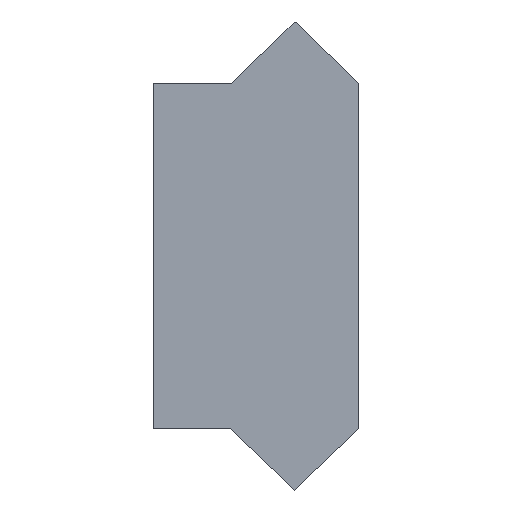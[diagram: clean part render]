
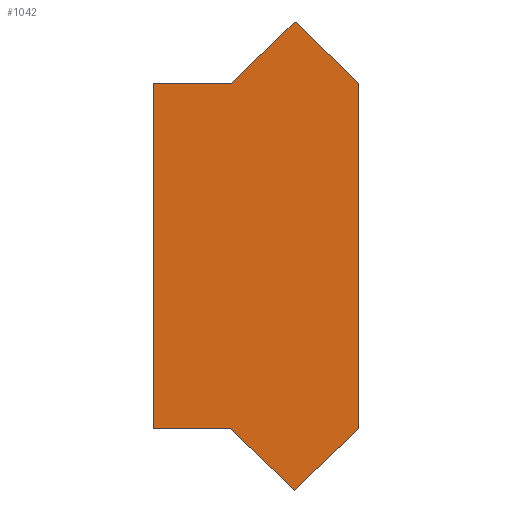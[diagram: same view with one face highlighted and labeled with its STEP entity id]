
A CAD part, front view. The second image highlights one B-rep face of the part: STEP entity #1042.
In plain terms, the highlighted planar face has unit normal (0, -1, 0).
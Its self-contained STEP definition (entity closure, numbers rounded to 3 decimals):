
#72=PLANE('',#1111);
#126=FACE_OUTER_BOUND('',#184,.T.);
#184=EDGE_LOOP('',(#977,#978,#979,#980,#981,#982,#983,#984));
#216=LINE('',#1477,#348);
#219=LINE('',#1482,#351);
#249=LINE('',#1544,#381);
#265=LINE('',#1577,#397);
#282=LINE('',#1607,#414);
#312=LINE('',#1666,#444);
#314=LINE('',#1670,#446);
#316=LINE('',#1673,#448);
#348=VECTOR('',#1196,10.);
#351=VECTOR('',#1201,10.);
#381=VECTOR('',#1243,10.);
#397=VECTOR('',#1269,10.);
#414=VECTOR('',#1300,10.);
#444=VECTOR('',#1370,10.);
#446=VECTOR('',#1374,10.);
#448=VECTOR('',#1378,10.);
#496=VERTEX_POINT('',#1475);
#497=VERTEX_POINT('',#1476);
#498=VERTEX_POINT('',#1481);
#523=VERTEX_POINT('',#1542);
#524=VERTEX_POINT('',#1543);
#536=VERTEX_POINT('',#1576);
#551=VERTEX_POINT('',#1665);
#552=VERTEX_POINT('',#1669);
#596=EDGE_CURVE('',#496,#497,#216,.T.);
#599=EDGE_CURVE('',#497,#498,#219,.T.);
#629=EDGE_CURVE('',#523,#524,#249,.T.);
#645=EDGE_CURVE('',#524,#536,#265,.T.);
#662=EDGE_CURVE('',#536,#498,#282,.T.);
#692=EDGE_CURVE('',#523,#551,#312,.T.);
#694=EDGE_CURVE('',#551,#552,#314,.T.);
#696=EDGE_CURVE('',#552,#496,#316,.T.);
#977=ORIENTED_EDGE('',*,*,#692,.T.);
#978=ORIENTED_EDGE('',*,*,#694,.T.);
#979=ORIENTED_EDGE('',*,*,#696,.T.);
#980=ORIENTED_EDGE('',*,*,#596,.T.);
#981=ORIENTED_EDGE('',*,*,#599,.T.);
#982=ORIENTED_EDGE('',*,*,#662,.F.);
#983=ORIENTED_EDGE('',*,*,#645,.F.);
#984=ORIENTED_EDGE('',*,*,#629,.F.);
#1042=ADVANCED_FACE('',(#126),#72,.T.);
#1111=AXIS2_PLACEMENT_3D('',#1674,#1379,#1380);
#1196=DIRECTION('',(1.,0.,0.));
#1201=DIRECTION('',(0.725,0.,-0.689));
#1243=DIRECTION('',(0.722,0.,-0.692));
#1269=DIRECTION('',(0.,0.,-1.));
#1300=DIRECTION('',(-0.726,0.,-0.688));
#1370=DIRECTION('',(-0.723,0.,-0.691));
#1374=DIRECTION('',(-1.,0.,0.));
#1378=DIRECTION('',(0.,0.,-1.));
#1379=DIRECTION('center_axis',(0.,-1.,0.));
#1380=DIRECTION('ref_axis',(0.,0.,-1.));
#1475=CARTESIAN_POINT('',(-71.601,-57.922,-11.679));
#1476=CARTESIAN_POINT('',(-68.111,-57.922,-11.679));
#1477=CARTESIAN_POINT('',(-69.271,-57.922,-11.679));
#1481=CARTESIAN_POINT('',(-65.199,-57.922,-14.448));
#1482=CARTESIAN_POINT('',(-69.76,-57.922,-10.111));
#1542=CARTESIAN_POINT('',(-65.169,-57.922,6.761));
#1543=CARTESIAN_POINT('',(-62.28,-57.922,3.993));
#1544=CARTESIAN_POINT('',(-58.365,-57.922,0.242));
#1576=CARTESIAN_POINT('',(-62.28,-57.922,-11.679));
#1577=CARTESIAN_POINT('',(-62.28,-57.922,-11.679));
#1607=CARTESIAN_POINT('',(-63.74,-57.922,-13.063));
#1665=CARTESIAN_POINT('',(-68.066,-57.922,3.993));
#1666=CARTESIAN_POINT('',(-68.28,-57.922,3.788));
#1669=CARTESIAN_POINT('',(-71.601,-57.922,3.993));
#1670=CARTESIAN_POINT('',(-67.503,-57.922,3.993));
#1673=CARTESIAN_POINT('',(-71.601,-57.922,0.075));
#1674=CARTESIAN_POINT('Origin',(-66.941,-57.922,-3.843));
